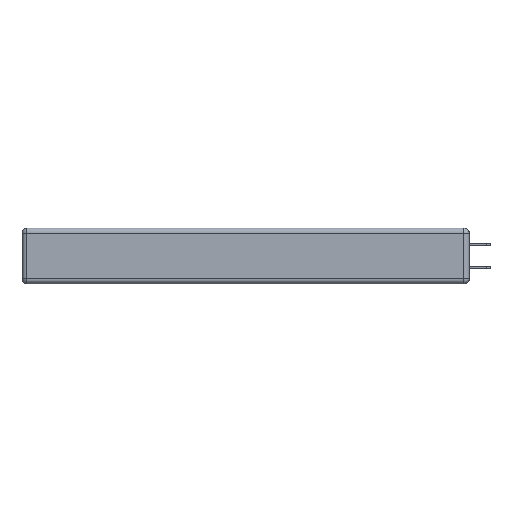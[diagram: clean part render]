
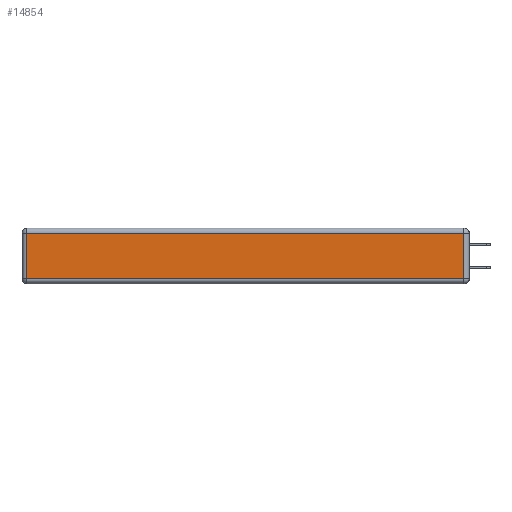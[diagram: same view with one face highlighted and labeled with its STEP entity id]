
A CAD part, left-side view. The second image highlights one B-rep face of the part: STEP entity #14854.
In plain terms, the highlighted planar face has unit normal (-1, 0, 0).
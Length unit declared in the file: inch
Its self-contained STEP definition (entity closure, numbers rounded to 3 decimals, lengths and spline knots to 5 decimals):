
#22 = CARTESIAN_POINT ( 'NONE',  ( 0., 0.03, -0.03 ) ) ;
#548 = LINE ( 'NONE', #15389, #2573 ) ;
#1087 = EDGE_CURVE ( 'NONE', #5056, #2449, #12704, .T. ) ;
#1467 = CARTESIAN_POINT ( 'NONE',  ( 0., 0., -0.343 ) ) ;
#1813 = DIRECTION ( 'NONE',  ( 0., 0., 1. ) ) ;
#1814 = CARTESIAN_POINT ( 'NONE',  ( 0., 2.75, -0.03 ) ) ;
#1869 = DIRECTION ( 'NONE',  ( 0., 1., 0. ) ) ;
#2416 = CARTESIAN_POINT ( 'NONE',  ( 0., 2.72, -0.03 ) ) ;
#2449 = VERTEX_POINT ( 'NONE', #13134 ) ;
#2506 = LINE ( 'NONE', #12201, #5299 ) ;
#2573 = VECTOR ( 'NONE', #15241, 39.37008 ) ;
#2695 = VERTEX_POINT ( 'NONE', #4181 ) ;
#3231 = EDGE_CURVE ( 'NONE', #3653, #5056, #3350, .T. ) ;
#3350 = LINE ( 'NONE', #1814, #13956 ) ;
#3653 = VERTEX_POINT ( 'NONE', #22 ) ;
#4181 = CARTESIAN_POINT ( 'NONE',  ( 0., 0.03, -0.313 ) ) ;
#4557 = ORIENTED_EDGE ( 'NONE', *, *, #8016, .T. ) ;
#5056 = VERTEX_POINT ( 'NONE', #2416 ) ;
#5299 = VECTOR ( 'NONE', #8677, 39.37008 ) ;
#5633 = EDGE_CURVE ( 'NONE', #2695, #3653, #2506, .T. ) ;
#5826 = ORIENTED_EDGE ( 'NONE', *, *, #3231, .T. ) ;
#8016 = EDGE_CURVE ( 'NONE', #2449, #2695, #548, .T. ) ;
#8661 = PLANE ( 'NONE',  #13158 ) ;
#8677 = DIRECTION ( 'NONE',  ( 0., 0., 1. ) ) ;
#9437 = DIRECTION ( 'NONE',  ( 0., 0., -1. ) ) ;
#9524 = VECTOR ( 'NONE', #9437, 39.37008 ) ;
#10482 = ORIENTED_EDGE ( 'NONE', *, *, #5633, .T. ) ;
#10694 = ORIENTED_EDGE ( 'NONE', *, *, #1087, .T. ) ;
#12201 = CARTESIAN_POINT ( 'NONE',  ( 0., 0.03, -0.343 ) ) ;
#12704 = LINE ( 'NONE', #13003, #9524 ) ;
#13003 = CARTESIAN_POINT ( 'NONE',  ( 0., 2.72, -0.343 ) ) ;
#13134 = CARTESIAN_POINT ( 'NONE',  ( 0., 2.72, -0.313 ) ) ;
#13158 = AXIS2_PLACEMENT_3D ( 'NONE', #1467, #14859, #1813 ) ;
#13956 = VECTOR ( 'NONE', #1869, 39.37008 ) ;
#14854 = ADVANCED_FACE ( 'NONE', ( #14953 ), #8661, .T. ) ;
#14859 = DIRECTION ( 'NONE',  ( -1., 0., 0. ) ) ;
#14953 = FACE_OUTER_BOUND ( 'NONE', #15358, .T. ) ;
#15241 = DIRECTION ( 'NONE',  ( 0., -1., 0. ) ) ;
#15358 = EDGE_LOOP ( 'NONE', ( #4557, #10482, #5826, #10694 ) ) ;
#15389 = CARTESIAN_POINT ( 'NONE',  ( 0., 0., -0.313 ) ) ;
